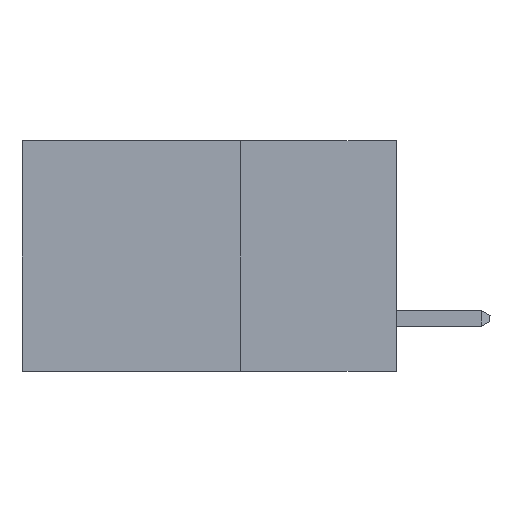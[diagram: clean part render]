
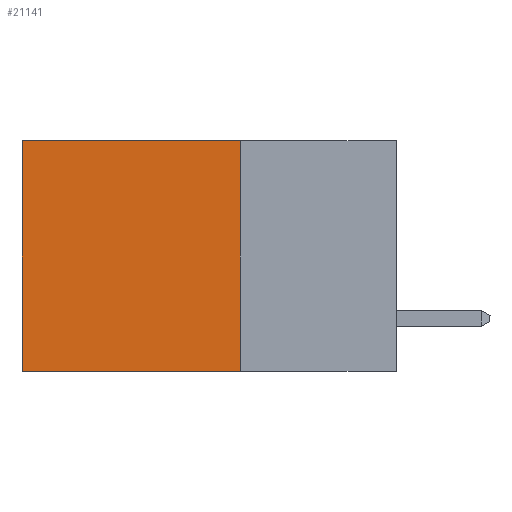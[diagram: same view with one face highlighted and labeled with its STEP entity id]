
A CAD part, left-side view. The second image highlights one B-rep face of the part: STEP entity #21141.
In plain terms, the highlighted planar face has unit normal (-1, 0, 0).
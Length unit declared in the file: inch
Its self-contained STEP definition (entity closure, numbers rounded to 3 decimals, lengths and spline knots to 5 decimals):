
#134 = VERTEX_POINT ( 'NONE', #13773 ) ;
#611 = LINE ( 'NONE', #2466, #14704 ) ;
#1149 = DIRECTION ( 'NONE',  ( 0., 0., -1. ) ) ;
#1832 = PLANE ( 'NONE',  #5562 ) ;
#2466 = CARTESIAN_POINT ( 'NONE',  ( 0.2615, 0.25, 0. ) ) ;
#2778 = LINE ( 'NONE', #21554, #16254 ) ;
#3630 = DIRECTION ( 'NONE',  ( 1., 0., 0. ) ) ;
#4283 = DIRECTION ( 'NONE',  ( 0., 1., 0. ) ) ;
#5562 = AXIS2_PLACEMENT_3D ( 'NONE', #10595, #3630, #15920 ) ;
#5648 = CARTESIAN_POINT ( 'NONE',  ( 0.2615, 0.6, 0. ) ) ;
#5839 = VECTOR ( 'NONE', #7870, 39.37008 ) ;
#5841 = EDGE_LOOP ( 'NONE', ( #7571, #9222, #11289, #22493 ) ) ;
#6093 = VERTEX_POINT ( 'NONE', #8245 ) ;
#6112 = CARTESIAN_POINT ( 'NONE',  ( 0.2615, 0.25, -0.37 ) ) ;
#6185 = LINE ( 'NONE', #13505, #7282 ) ;
#7282 = VECTOR ( 'NONE', #1149, 39.37008 ) ;
#7571 = ORIENTED_EDGE ( 'NONE', *, *, #21343, .T. ) ;
#7870 = DIRECTION ( 'NONE',  ( 0., 1., 0. ) ) ;
#8245 = CARTESIAN_POINT ( 'NONE',  ( 0.2615, 0.25, -0.37 ) ) ;
#9222 = ORIENTED_EDGE ( 'NONE', *, *, #21380, .F. ) ;
#10595 = CARTESIAN_POINT ( 'NONE',  ( 0.2615, 0.25, -0.37 ) ) ;
#11273 = DIRECTION ( 'NONE',  ( 0., 0., -1. ) ) ;
#11289 = ORIENTED_EDGE ( 'NONE', *, *, #16228, .F. ) ;
#13504 = CARTESIAN_POINT ( 'NONE',  ( 0.2615, 0.25, 0. ) ) ;
#13505 = CARTESIAN_POINT ( 'NONE',  ( 0.2615, 0.25, -0.37 ) ) ;
#13773 = CARTESIAN_POINT ( 'NONE',  ( 0.2615, 0.6, -0.37 ) ) ;
#14373 = VERTEX_POINT ( 'NONE', #13504 ) ;
#14704 = VECTOR ( 'NONE', #4283, 39.37008 ) ;
#15920 = DIRECTION ( 'NONE',  ( 0., 0., -1. ) ) ;
#16070 = EDGE_CURVE ( 'NONE', #14373, #21225, #611, .T. ) ;
#16228 = EDGE_CURVE ( 'NONE', #14373, #6093, #6185, .T. ) ;
#16254 = VECTOR ( 'NONE', #11273, 39.37008 ) ;
#19734 = LINE ( 'NONE', #6112, #5839 ) ;
#21141 = ADVANCED_FACE ( 'NONE', ( #22195 ), #1832, .F. ) ;
#21225 = VERTEX_POINT ( 'NONE', #5648 ) ;
#21343 = EDGE_CURVE ( 'NONE', #21225, #134, #2778, .T. ) ;
#21380 = EDGE_CURVE ( 'NONE', #6093, #134, #19734, .T. ) ;
#21554 = CARTESIAN_POINT ( 'NONE',  ( 0.2615, 0.6, -0.37 ) ) ;
#22195 = FACE_OUTER_BOUND ( 'NONE', #5841, .T. ) ;
#22493 = ORIENTED_EDGE ( 'NONE', *, *, #16070, .T. ) ;
